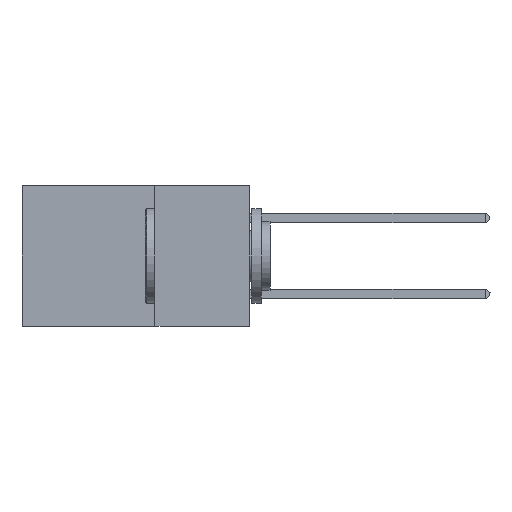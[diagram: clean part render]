
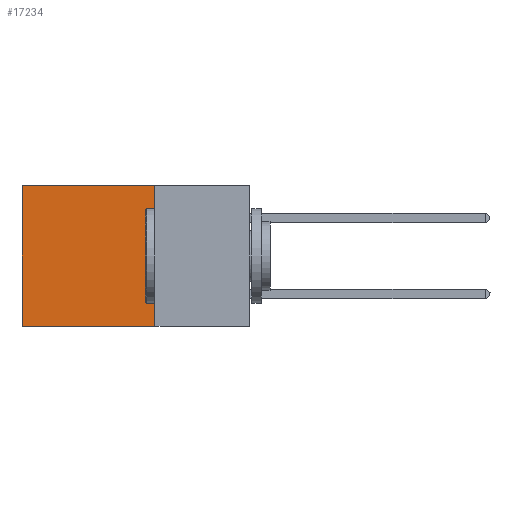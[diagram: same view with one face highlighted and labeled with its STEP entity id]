
A CAD part, left-side view. The second image highlights one B-rep face of the part: STEP entity #17234.
In plain terms, the highlighted planar face has unit normal (-1, 0, 0).
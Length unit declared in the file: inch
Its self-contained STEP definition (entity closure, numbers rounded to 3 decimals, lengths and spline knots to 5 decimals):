
#344 = VECTOR ( 'NONE', #27561, 39.37008 ) ;
#636 = VERTEX_POINT ( 'NONE', #14954 ) ;
#687 = EDGE_LOOP ( 'NONE', ( #13849, #22058, #10856, #17471 ) ) ;
#798 = LINE ( 'NONE', #24061, #22298 ) ;
#1051 = CARTESIAN_POINT ( 'NONE',  ( 0.2875, 0.25, 0. ) ) ;
#1181 = CARTESIAN_POINT ( 'NONE',  ( 0.2875, 0.25, 0. ) ) ;
#1235 = VECTOR ( 'NONE', #6571, 39.37008 ) ;
#1627 = EDGE_CURVE ( 'NONE', #636, #25353, #7957, .T. ) ;
#4338 = VECTOR ( 'NONE', #31275, 39.37008 ) ;
#6571 = DIRECTION ( 'NONE',  ( 0., 1., 0. ) ) ;
#7692 = CARTESIAN_POINT ( 'NONE',  ( 0.2875, 0.25, 0. ) ) ;
#7696 = EDGE_CURVE ( 'NONE', #26693, #25353, #7882, .T. ) ;
#7882 = LINE ( 'NONE', #19849, #344 ) ;
#7957 = LINE ( 'NONE', #24465, #1235 ) ;
#9443 = PLANE ( 'NONE',  #9658 ) ;
#9658 = AXIS2_PLACEMENT_3D ( 'NONE', #7692, #32900, #25357 ) ;
#10856 = ORIENTED_EDGE ( 'NONE', *, *, #31734, .F. ) ;
#13849 = ORIENTED_EDGE ( 'NONE', *, *, #7696, .T. ) ;
#14296 = LINE ( 'NONE', #1051, #4338 ) ;
#14495 = EDGE_CURVE ( 'NONE', #30300, #26693, #14296, .T. ) ;
#14954 = CARTESIAN_POINT ( 'NONE',  ( 0.2875, 0.25, -0.37 ) ) ;
#17234 = ADVANCED_FACE ( 'NONE', ( #32921 ), #9443, .F. ) ;
#17471 = ORIENTED_EDGE ( 'NONE', *, *, #14495, .T. ) ;
#17670 = CARTESIAN_POINT ( 'NONE',  ( 0.2875, 0.6, 0. ) ) ;
#19008 = DIRECTION ( 'NONE',  ( 0., 0., -1. ) ) ;
#19849 = CARTESIAN_POINT ( 'NONE',  ( 0.2875, 0.6, 0. ) ) ;
#22058 = ORIENTED_EDGE ( 'NONE', *, *, #1627, .F. ) ;
#22298 = VECTOR ( 'NONE', #19008, 39.37008 ) ;
#24061 = CARTESIAN_POINT ( 'NONE',  ( 0.2875, 0.25, 0. ) ) ;
#24465 = CARTESIAN_POINT ( 'NONE',  ( 0.2875, 0.25, -0.37 ) ) ;
#24533 = CARTESIAN_POINT ( 'NONE',  ( 0.2875, 0.6, -0.37 ) ) ;
#25353 = VERTEX_POINT ( 'NONE', #24533 ) ;
#25357 = DIRECTION ( 'NONE',  ( 0., 0., -1. ) ) ;
#26693 = VERTEX_POINT ( 'NONE', #17670 ) ;
#27561 = DIRECTION ( 'NONE',  ( 0., 0., -1. ) ) ;
#30300 = VERTEX_POINT ( 'NONE', #1181 ) ;
#31275 = DIRECTION ( 'NONE',  ( 0., 1., 0. ) ) ;
#31734 = EDGE_CURVE ( 'NONE', #30300, #636, #798, .T. ) ;
#32900 = DIRECTION ( 'NONE',  ( 1., 0., 0. ) ) ;
#32921 = FACE_OUTER_BOUND ( 'NONE', #687, .T. ) ;
